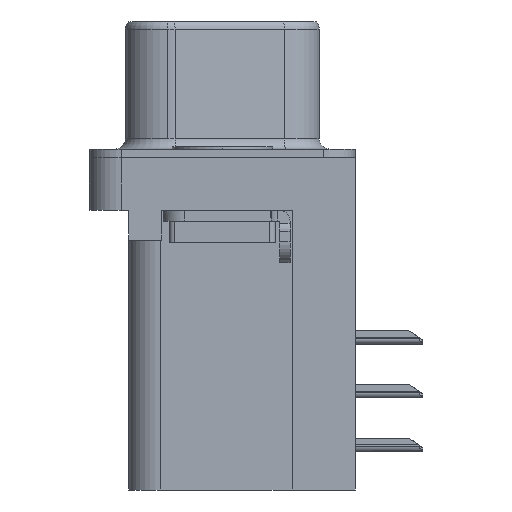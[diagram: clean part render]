
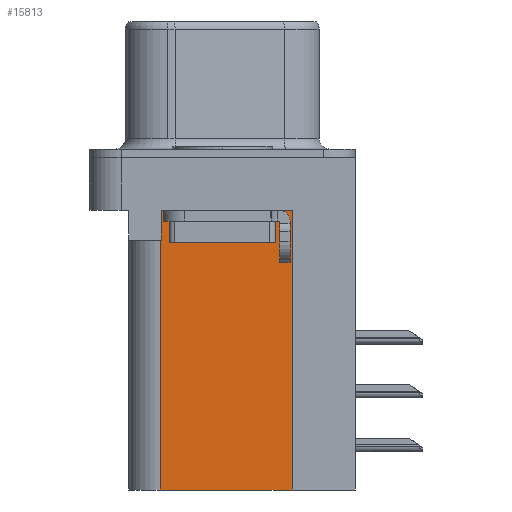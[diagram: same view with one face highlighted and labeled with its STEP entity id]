
A CAD part, left-side view. The second image highlights one B-rep face of the part: STEP entity #15813.
In plain terms, the highlighted planar face has unit normal (-1, 0, 0).
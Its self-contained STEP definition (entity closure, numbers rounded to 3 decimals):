
#552 = CARTESIAN_POINT ( 'NONE',  ( 3.7, -3.295, -15.7 ) ) ;
#814 = DIRECTION ( 'NONE',  ( 0., 0., -1. ) ) ;
#909 = LINE ( 'NONE', #2190, #6517 ) ;
#1048 = CARTESIAN_POINT ( 'NONE',  ( 3.7, 0., -3.9 ) ) ;
#1122 = DIRECTION ( 'NONE',  ( 0., 1., 0. ) ) ;
#1507 = CARTESIAN_POINT ( 'NONE',  ( 3.7, 2.925, -15.7 ) ) ;
#1746 = EDGE_CURVE ( 'NONE', #3151, #16638, #14211, .T. ) ;
#2190 = CARTESIAN_POINT ( 'NONE',  ( 3.7, -3.295, -2.5 ) ) ;
#2349 = VECTOR ( 'NONE', #3592, 1000. ) ;
#2516 = ORIENTED_EDGE ( 'NONE', *, *, #6306, .T. ) ;
#2588 = VECTOR ( 'NONE', #1122, 1000. ) ;
#2945 = CARTESIAN_POINT ( 'NONE',  ( 3.7, 2.895, -3.9 ) ) ;
#3031 = EDGE_LOOP ( 'NONE', ( #2516, #15827, #4323, #6337, #25542, #24165 ) ) ;
#3151 = VERTEX_POINT ( 'NONE', #19958 ) ;
#3411 = EDGE_CURVE ( 'NONE', #17662, #16638, #18738, .T. ) ;
#3592 = DIRECTION ( 'NONE',  ( 0., 0., 1. ) ) ;
#4323 = ORIENTED_EDGE ( 'NONE', *, *, #3411, .T. ) ;
#4826 = PLANE ( 'NONE',  #15966 ) ;
#4975 = EDGE_CURVE ( 'NONE', #12105, #3151, #16658, .T. ) ;
#6306 = EDGE_CURVE ( 'NONE', #13619, #17481, #909, .T. ) ;
#6337 = ORIENTED_EDGE ( 'NONE', *, *, #1746, .F. ) ;
#6389 = VECTOR ( 'NONE', #814, 1000. ) ;
#6517 = VECTOR ( 'NONE', #21023, 1000. ) ;
#8132 = CARTESIAN_POINT ( 'NONE',  ( 3.7, -3.295, -15.7 ) ) ;
#8323 = EDGE_CURVE ( 'NONE', #17481, #17662, #17555, .T. ) ;
#9139 = VECTOR ( 'NONE', #13898, 1000. ) ;
#10404 = VECTOR ( 'NONE', #16763, 1000. ) ;
#10672 = CARTESIAN_POINT ( 'NONE',  ( 3.7, 2.895, -2.5 ) ) ;
#11130 = DIRECTION ( 'NONE',  ( 1., 0., 0. ) ) ;
#12105 = VERTEX_POINT ( 'NONE', #8132 ) ;
#12539 = CARTESIAN_POINT ( 'NONE',  ( 3.7, -3.295, -15.7 ) ) ;
#12576 = EDGE_CURVE ( 'NONE', #12105, #13619, #23257, .T. ) ;
#13619 = VERTEX_POINT ( 'NONE', #21543 ) ;
#13898 = DIRECTION ( 'NONE',  ( 0., 0., 1. ) ) ;
#14211 = LINE ( 'NONE', #1507, #2349 ) ;
#15513 = CARTESIAN_POINT ( 'NONE',  ( 3.7, 2.895, -3.9 ) ) ;
#15813 = ADVANCED_FACE ( 'NONE', ( #22420 ), #4826, .F. ) ;
#15827 = ORIENTED_EDGE ( 'NONE', *, *, #8323, .T. ) ;
#15956 = CARTESIAN_POINT ( 'NONE',  ( 3.7, 2.925, -3.9 ) ) ;
#15966 = AXIS2_PLACEMENT_3D ( 'NONE', #552, #11130, #25830 ) ;
#16638 = VERTEX_POINT ( 'NONE', #15956 ) ;
#16658 = LINE ( 'NONE', #12539, #10404 ) ;
#16763 = DIRECTION ( 'NONE',  ( 0., 1., 0. ) ) ;
#17481 = VERTEX_POINT ( 'NONE', #10672 ) ;
#17555 = LINE ( 'NONE', #15513, #6389 ) ;
#17662 = VERTEX_POINT ( 'NONE', #2945 ) ;
#18738 = LINE ( 'NONE', #1048, #2588 ) ;
#19958 = CARTESIAN_POINT ( 'NONE',  ( 3.7, 2.925, -15.7 ) ) ;
#21023 = DIRECTION ( 'NONE',  ( 0., 1., 0. ) ) ;
#21543 = CARTESIAN_POINT ( 'NONE',  ( 3.7, -3.295, -2.5 ) ) ;
#22420 = FACE_OUTER_BOUND ( 'NONE', #3031, .T. ) ;
#23257 = LINE ( 'NONE', #26437, #9139 ) ;
#24165 = ORIENTED_EDGE ( 'NONE', *, *, #12576, .T. ) ;
#25542 = ORIENTED_EDGE ( 'NONE', *, *, #4975, .F. ) ;
#25830 = DIRECTION ( 'NONE',  ( 0., 0., -1. ) ) ;
#26437 = CARTESIAN_POINT ( 'NONE',  ( 3.7, -3.295, -15.7 ) ) ;
